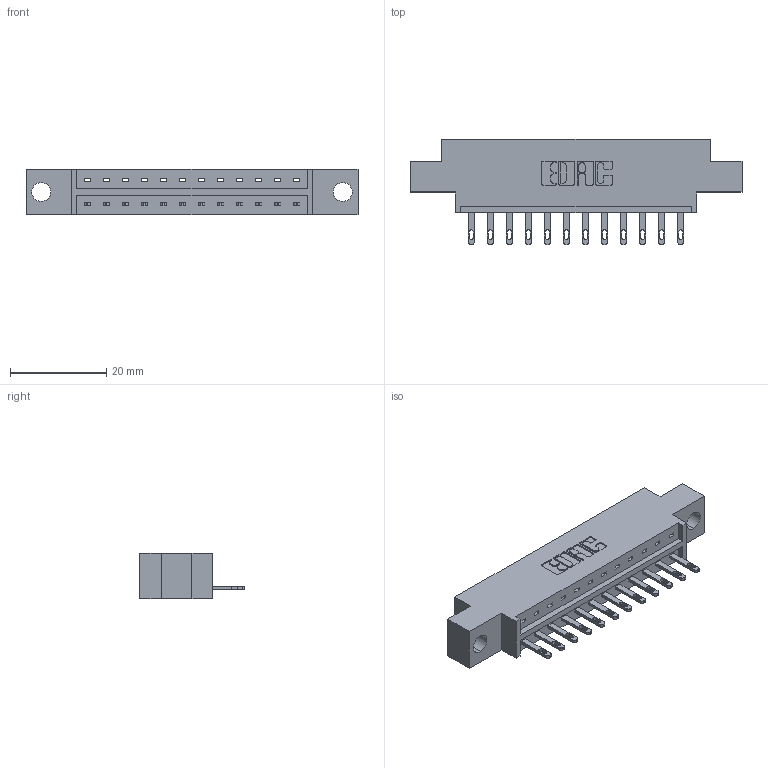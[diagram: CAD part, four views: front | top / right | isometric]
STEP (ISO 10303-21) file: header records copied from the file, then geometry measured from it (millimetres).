
FILE_DESCRIPTION (( 'STEP AP203' ), '1' );
FILE_NAME ('333-012-500-604.STEP', '2018-07-31T23:49:04', ( '' ), ( '' ), 'SwSTEP 2.0', 'SolidWorks 2016', '' );
FILE_SCHEMA (( 'CONFIG_CONTROL_DESIGN' ));
Length unit declared in the file: inch
Products named in the file (3): 333 Part_Offset - .156 Dia - TH; 345-292-001_345-293-100; 333-012-500-604
Assembly tree (13 placements, depth 2):
  333-012-500-604
    333 Part_Offset - .156 Dia - TH
    345-292-001_345-293-100  x12
Bounding box: 69.09 x 21.85 x 9.4 mm (x, y, z)
Volume: 6386 mm3; surface area: 6735.6 mm2
Topology: 13 solids, 13 shells, 766 faces, 2339 edges, 1558 vertices
Faces by surface type: plane 506, cylinder 260
Entity records: 11281 total; most frequent: CARTESIAN_POINT 1958, ORIENTED_EDGE 1906, DIRECTION 1713, EDGE_CURVE 953, LINE 821, VECTOR 821, VERTEX_POINT 634, AXIS2_PLACEMENT_3D 446
